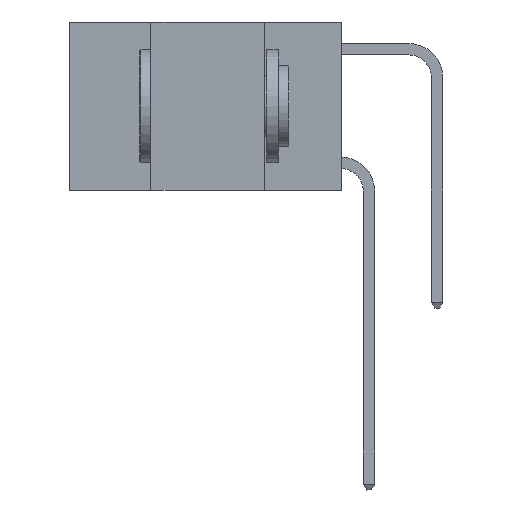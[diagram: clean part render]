
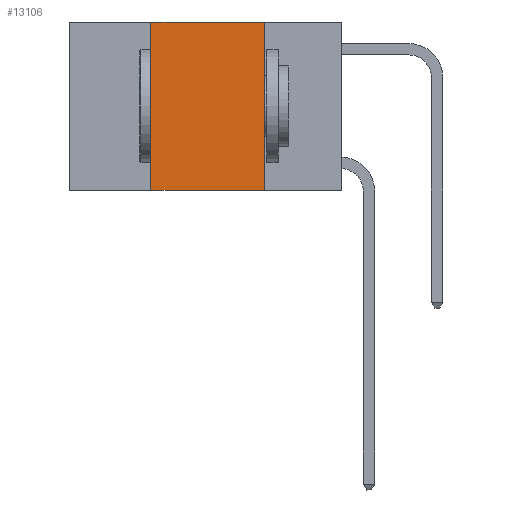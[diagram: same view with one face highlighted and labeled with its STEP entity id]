
A CAD part, left-side view. The second image highlights one B-rep face of the part: STEP entity #13106.
In plain terms, the highlighted planar face has unit normal (-1, 0, 0).
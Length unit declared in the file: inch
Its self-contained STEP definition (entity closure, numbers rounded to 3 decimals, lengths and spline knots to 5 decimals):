
#456 = LINE ( 'NONE', #1629, #9276 ) ;
#1629 = CARTESIAN_POINT ( 'NONE',  ( 0., 0.6, -0.37 ) ) ;
#2113 = DIRECTION ( 'NONE',  ( 0., -1., 0. ) ) ;
#2895 = VERTEX_POINT ( 'NONE', #5786 ) ;
#3454 = LINE ( 'NONE', #15370, #16356 ) ;
#3973 = VECTOR ( 'NONE', #12445, 39.37008 ) ;
#4243 = CARTESIAN_POINT ( 'NONE',  ( 0., 0.17, -0.37 ) ) ;
#4474 = ORIENTED_EDGE ( 'NONE', *, *, #4785, .F. ) ;
#4495 = CARTESIAN_POINT ( 'NONE',  ( 0., 0.42, -0.37 ) ) ;
#4785 = EDGE_CURVE ( 'NONE', #11999, #2895, #16469, .T. ) ;
#5786 = CARTESIAN_POINT ( 'NONE',  ( 0., 0.42, 0. ) ) ;
#5869 = FACE_OUTER_BOUND ( 'NONE', #10370, .T. ) ;
#7065 = CARTESIAN_POINT ( 'NONE',  ( 0., 0.17, 0. ) ) ;
#7266 = VERTEX_POINT ( 'NONE', #4243 ) ;
#9276 = VECTOR ( 'NONE', #11366, 39.37008 ) ;
#9932 = DIRECTION ( 'NONE',  ( 1., 0., 0. ) ) ;
#10066 = CARTESIAN_POINT ( 'NONE',  ( 0., 0.17, 0. ) ) ;
#10370 = EDGE_LOOP ( 'NONE', ( #16550, #13320, #4474, #12515 ) ) ;
#10521 = EDGE_CURVE ( 'NONE', #11999, #7266, #456, .T. ) ;
#11248 = PLANE ( 'NONE',  #11539 ) ;
#11366 = DIRECTION ( 'NONE',  ( 0., -1., 0. ) ) ;
#11539 = AXIS2_PLACEMENT_3D ( 'NONE', #16611, #9932, #13974 ) ;
#11999 = VERTEX_POINT ( 'NONE', #4495 ) ;
#12099 = LINE ( 'NONE', #7065, #3973 ) ;
#12445 = DIRECTION ( 'NONE',  ( 0., 0., -1. ) ) ;
#12515 = ORIENTED_EDGE ( 'NONE', *, *, #10521, .T. ) ;
#12516 = CARTESIAN_POINT ( 'NONE',  ( 0., 0.42, 0. ) ) ;
#13106 = ADVANCED_FACE ( 'NONE', ( #5869 ), #11248, .F. ) ;
#13320 = ORIENTED_EDGE ( 'NONE', *, *, #14467, .F. ) ;
#13974 = DIRECTION ( 'NONE',  ( 0., 0., -1. ) ) ;
#14467 = EDGE_CURVE ( 'NONE', #2895, #16689, #3454, .T. ) ;
#14981 = DIRECTION ( 'NONE',  ( 0., 0., 1. ) ) ;
#15229 = EDGE_CURVE ( 'NONE', #16689, #7266, #12099, .T. ) ;
#15370 = CARTESIAN_POINT ( 'NONE',  ( 0., 0.6, 0. ) ) ;
#16356 = VECTOR ( 'NONE', #2113, 39.37008 ) ;
#16469 = LINE ( 'NONE', #12516, #17023 ) ;
#16550 = ORIENTED_EDGE ( 'NONE', *, *, #15229, .F. ) ;
#16611 = CARTESIAN_POINT ( 'NONE',  ( 0., 0.6, 0. ) ) ;
#16689 = VERTEX_POINT ( 'NONE', #10066 ) ;
#17023 = VECTOR ( 'NONE', #14981, 39.37008 ) ;
